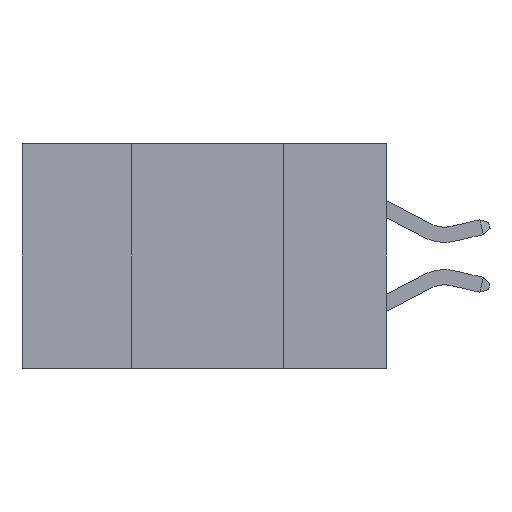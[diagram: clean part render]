
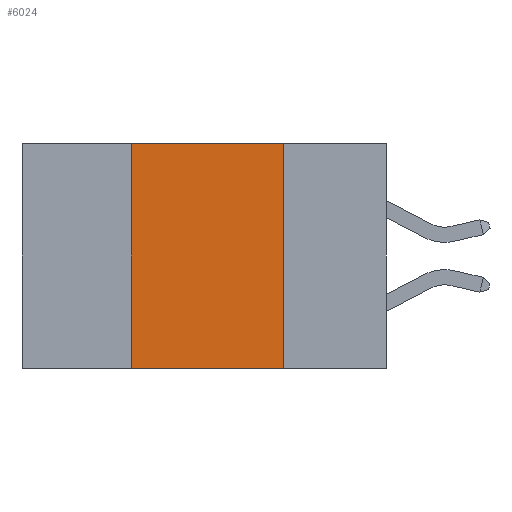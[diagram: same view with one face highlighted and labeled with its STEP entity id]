
A CAD part, left-side view. The second image highlights one B-rep face of the part: STEP entity #6024.
In plain terms, the highlighted planar face has unit normal (-1, 0, 0).
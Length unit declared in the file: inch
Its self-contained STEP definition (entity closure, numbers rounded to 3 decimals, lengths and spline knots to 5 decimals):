
#369 = DIRECTION ( 'NONE',  ( 0., -1., 0. ) ) ;
#464 = PLANE ( 'NONE',  #10824 ) ;
#579 = CARTESIAN_POINT ( 'NONE',  ( 0., 0.6, 0. ) ) ;
#911 = VERTEX_POINT ( 'NONE', #5490 ) ;
#2278 = DIRECTION ( 'NONE',  ( 0., 0., 1. ) ) ;
#2461 = FACE_OUTER_BOUND ( 'NONE', #7498, .T. ) ;
#2481 = VECTOR ( 'NONE', #5346, 39.37008 ) ;
#2834 = EDGE_CURVE ( 'NONE', #911, #6327, #12394, .T. ) ;
#3402 = CARTESIAN_POINT ( 'NONE',  ( 0., 0.17, -0.37 ) ) ;
#3772 = LINE ( 'NONE', #11516, #5081 ) ;
#4162 = LINE ( 'NONE', #9341, #2481 ) ;
#4795 = ORIENTED_EDGE ( 'NONE', *, *, #13973, .F. ) ;
#5049 = VECTOR ( 'NONE', #2278, 39.37008 ) ;
#5081 = VECTOR ( 'NONE', #369, 39.37008 ) ;
#5119 = ORIENTED_EDGE ( 'NONE', *, *, #10707, .T. ) ;
#5346 = DIRECTION ( 'NONE',  ( 0., 0., -1. ) ) ;
#5490 = CARTESIAN_POINT ( 'NONE',  ( 0., 0.42, -0.37 ) ) ;
#5801 = DIRECTION ( 'NONE',  ( 1., 0., 0. ) ) ;
#6024 = ADVANCED_FACE ( 'NONE', ( #2461 ), #464, .F. ) ;
#6327 = VERTEX_POINT ( 'NONE', #7647 ) ;
#6466 = CARTESIAN_POINT ( 'NONE',  ( 0., 0.17, 0. ) ) ;
#6871 = CARTESIAN_POINT ( 'NONE',  ( 0., 0.42, -0.37 ) ) ;
#6985 = CARTESIAN_POINT ( 'NONE',  ( 0., 0.6, 0. ) ) ;
#7038 = ORIENTED_EDGE ( 'NONE', *, *, #11684, .F. ) ;
#7498 = EDGE_LOOP ( 'NONE', ( #7038, #4795, #12825, #5119 ) ) ;
#7647 = CARTESIAN_POINT ( 'NONE',  ( 0., 0.42, 0. ) ) ;
#8274 = LINE ( 'NONE', #579, #14301 ) ;
#8800 = VERTEX_POINT ( 'NONE', #6466 ) ;
#9327 = DIRECTION ( 'NONE',  ( 0., 0., -1. ) ) ;
#9341 = CARTESIAN_POINT ( 'NONE',  ( 0., 0.17, -0.37 ) ) ;
#10620 = VERTEX_POINT ( 'NONE', #3402 ) ;
#10707 = EDGE_CURVE ( 'NONE', #911, #10620, #3772, .T. ) ;
#10824 = AXIS2_PLACEMENT_3D ( 'NONE', #6985, #5801, #9327 ) ;
#11516 = CARTESIAN_POINT ( 'NONE',  ( 0., 0.6, -0.37 ) ) ;
#11579 = DIRECTION ( 'NONE',  ( 0., -1., 0. ) ) ;
#11684 = EDGE_CURVE ( 'NONE', #8800, #10620, #4162, .T. ) ;
#12394 = LINE ( 'NONE', #6871, #5049 ) ;
#12825 = ORIENTED_EDGE ( 'NONE', *, *, #2834, .F. ) ;
#13973 = EDGE_CURVE ( 'NONE', #6327, #8800, #8274, .T. ) ;
#14301 = VECTOR ( 'NONE', #11579, 39.37008 ) ;
